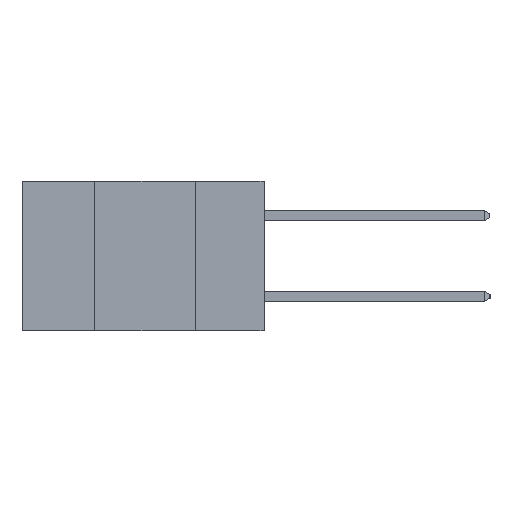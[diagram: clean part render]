
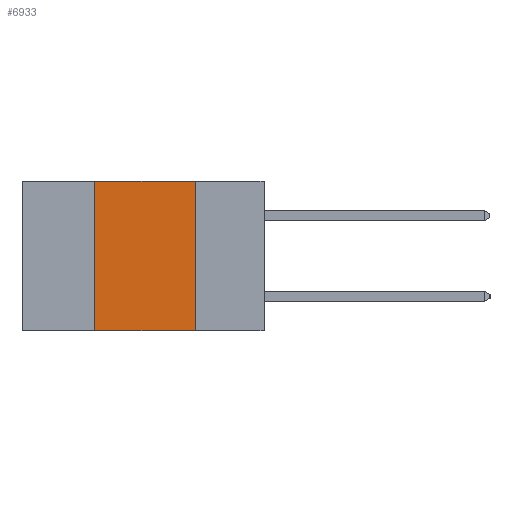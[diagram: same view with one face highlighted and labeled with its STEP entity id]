
A CAD part, left-side view. The second image highlights one B-rep face of the part: STEP entity #6933.
In plain terms, the highlighted planar face has unit normal (-1, 0, 0).
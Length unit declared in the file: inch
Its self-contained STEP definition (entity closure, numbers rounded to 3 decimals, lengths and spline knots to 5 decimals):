
#561 = LINE ( 'NONE', #5846, #6236 ) ;
#653 = VECTOR ( 'NONE', #6506, 39.37008 ) ;
#1076 = EDGE_CURVE ( 'NONE', #3683, #3738, #561, .T. ) ;
#1230 = VERTEX_POINT ( 'NONE', #2666 ) ;
#1998 = DIRECTION ( 'NONE',  ( 0., -1., 0. ) ) ;
#2132 = CARTESIAN_POINT ( 'NONE',  ( 0., 0.17, -0.37 ) ) ;
#2149 = DIRECTION ( 'NONE',  ( 0., 0., -1. ) ) ;
#2573 = PLANE ( 'NONE',  #7411 ) ;
#2666 = CARTESIAN_POINT ( 'NONE',  ( 0., 0.42, -0.37 ) ) ;
#2769 = LINE ( 'NONE', #6484, #653 ) ;
#3269 = VERTEX_POINT ( 'NONE', #6932 ) ;
#3378 = EDGE_CURVE ( 'NONE', #1230, #3269, #2769, .T. ) ;
#3506 = EDGE_LOOP ( 'NONE', ( #7100, #7092, #7055, #8042 ) ) ;
#3550 = CARTESIAN_POINT ( 'NONE',  ( 0., 0.42, -0.37 ) ) ;
#3683 = VERTEX_POINT ( 'NONE', #5149 ) ;
#3738 = VERTEX_POINT ( 'NONE', #4829 ) ;
#4157 = DIRECTION ( 'NONE',  ( 1., 0., 0. ) ) ;
#4330 = EDGE_CURVE ( 'NONE', #3738, #3269, #8490, .T. ) ;
#4574 = FACE_OUTER_BOUND ( 'NONE', #3506, .T. ) ;
#4829 = CARTESIAN_POINT ( 'NONE',  ( 0., 0.17, 0. ) ) ;
#5149 = CARTESIAN_POINT ( 'NONE',  ( 0., 0.42, 0. ) ) ;
#5514 = LINE ( 'NONE', #3550, #7178 ) ;
#5846 = CARTESIAN_POINT ( 'NONE',  ( 0., 0.6, 0. ) ) ;
#6236 = VECTOR ( 'NONE', #1998, 39.37008 ) ;
#6465 = EDGE_CURVE ( 'NONE', #1230, #3683, #5514, .T. ) ;
#6484 = CARTESIAN_POINT ( 'NONE',  ( 0., 0.6, -0.37 ) ) ;
#6506 = DIRECTION ( 'NONE',  ( 0., -1., 0. ) ) ;
#6524 = VECTOR ( 'NONE', #2149, 39.37008 ) ;
#6932 = CARTESIAN_POINT ( 'NONE',  ( 0., 0.17, -0.37 ) ) ;
#6933 = ADVANCED_FACE ( 'NONE', ( #4574 ), #2573, .F. ) ;
#7055 = ORIENTED_EDGE ( 'NONE', *, *, #6465, .F. ) ;
#7092 = ORIENTED_EDGE ( 'NONE', *, *, #1076, .F. ) ;
#7100 = ORIENTED_EDGE ( 'NONE', *, *, #4330, .F. ) ;
#7178 = VECTOR ( 'NONE', #7994, 39.37008 ) ;
#7411 = AXIS2_PLACEMENT_3D ( 'NONE', #8593, #4157, #9333 ) ;
#7994 = DIRECTION ( 'NONE',  ( 0., 0., 1. ) ) ;
#8042 = ORIENTED_EDGE ( 'NONE', *, *, #3378, .T. ) ;
#8490 = LINE ( 'NONE', #2132, #6524 ) ;
#8593 = CARTESIAN_POINT ( 'NONE',  ( 0., 0.6, 0. ) ) ;
#9333 = DIRECTION ( 'NONE',  ( 0., 0., -1. ) ) ;
